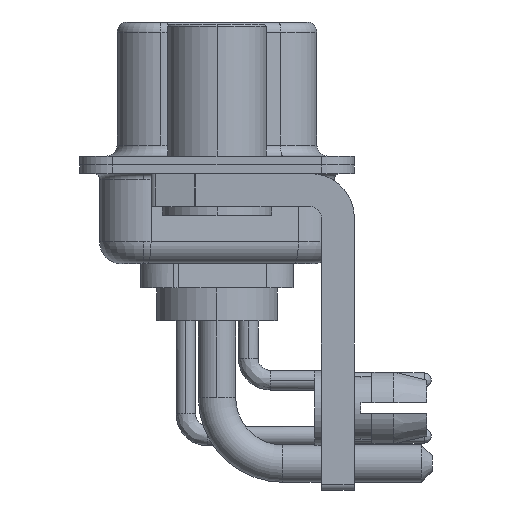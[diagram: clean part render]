
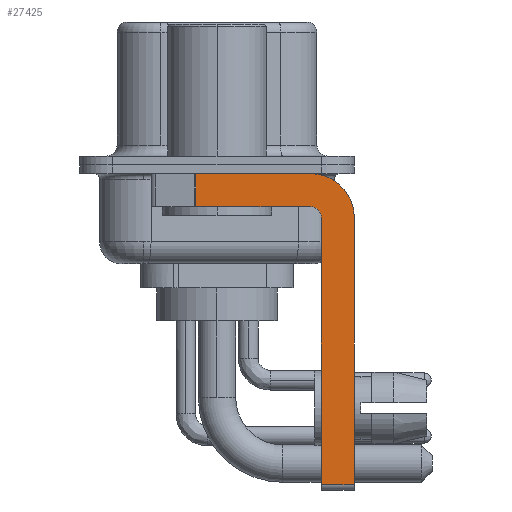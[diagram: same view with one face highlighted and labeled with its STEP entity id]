
A CAD part, left-side view. The second image highlights one B-rep face of the part: STEP entity #27425.
In plain terms, the highlighted planar face has unit normal (-1, 0, 0).
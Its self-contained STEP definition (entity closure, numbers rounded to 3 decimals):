
#953 = CARTESIAN_POINT ( 'NONE',  ( -2.9, -6.25, -2.4 ) ) ;
#1040 = EDGE_CURVE ( 'NONE', #17544, #20139, #19166, .T. ) ;
#1058 = VERTEX_POINT ( 'NONE', #6571 ) ;
#1455 = VERTEX_POINT ( 'NONE', #2155 ) ;
#1502 = LINE ( 'NONE', #8292, #12081 ) ;
#1587 = FACE_OUTER_BOUND ( 'NONE', #15525, .T. ) ;
#2068 = ORIENTED_EDGE ( 'NONE', *, *, #6072, .F. ) ;
#2155 = CARTESIAN_POINT ( 'NONE',  ( -2.9, -6.25, -2.4 ) ) ;
#2426 = EDGE_CURVE ( 'NONE', #4631, #17544, #14822, .T. ) ;
#2539 = CARTESIAN_POINT ( 'NONE',  ( -2.9, 3., -0.4 ) ) ;
#2830 = AXIS2_PLACEMENT_3D ( 'NONE', #15882, #17999, #25402 ) ;
#3077 = LINE ( 'NONE', #23118, #5850 ) ;
#3378 = EDGE_CURVE ( 'NONE', #4631, #26459, #1502, .T. ) ;
#3731 = CARTESIAN_POINT ( 'NONE',  ( -2.9, 0.978, -0.4 ) ) ;
#4164 = DIRECTION ( 'NONE',  ( 1., 0., 0. ) ) ;
#4443 = DIRECTION ( 'NONE',  ( 0., 0., -1. ) ) ;
#4631 = VERTEX_POINT ( 'NONE', #29277 ) ;
#5850 = VECTOR ( 'NONE', #9849, 1000. ) ;
#6072 = EDGE_CURVE ( 'NONE', #20139, #6119, #21003, .T. ) ;
#6119 = VERTEX_POINT ( 'NONE', #27779 ) ;
#6432 = CARTESIAN_POINT ( 'NONE',  ( -2.9, -4.25, -2.4 ) ) ;
#6571 = CARTESIAN_POINT ( 'NONE',  ( -2.9, -4.25, -0.4 ) ) ;
#6691 = CARTESIAN_POINT ( 'NONE',  ( -2.9, -4.75, -2.4 ) ) ;
#6985 = ORIENTED_EDGE ( 'NONE', *, *, #3378, .T. ) ;
#8292 = CARTESIAN_POINT ( 'NONE',  ( -2.9, -4.25, -14.55 ) ) ;
#9143 = ORIENTED_EDGE ( 'NONE', *, *, #14889, .T. ) ;
#9465 = DIRECTION ( 'NONE',  ( 0., -1., 0. ) ) ;
#9836 = ORIENTED_EDGE ( 'NONE', *, *, #1040, .F. ) ;
#9849 = DIRECTION ( 'NONE',  ( 0., 0., -1. ) ) ;
#9856 = CARTESIAN_POINT ( 'NONE',  ( -2.9, -4.25, -1.9 ) ) ;
#10759 = DIRECTION ( 'NONE',  ( 0., 0., 1. ) ) ;
#11224 = ORIENTED_EDGE ( 'NONE', *, *, #2426, .F. ) ;
#11385 = DIRECTION ( 'NONE',  ( 0., 0., -1. ) ) ;
#12081 = VECTOR ( 'NONE', #19882, 1000. ) ;
#12334 = ORIENTED_EDGE ( 'NONE', *, *, #12372, .F. ) ;
#12372 = EDGE_CURVE ( 'NONE', #18295, #1058, #26037, .T. ) ;
#12521 = CARTESIAN_POINT ( 'NONE',  ( -2.9, -4.25, -1.9 ) ) ;
#14790 = DIRECTION ( 'NONE',  ( 0., 0., -1. ) ) ;
#14822 = LINE ( 'NONE', #29266, #29324 ) ;
#14889 = EDGE_CURVE ( 'NONE', #18295, #6119, #3077, .T. ) ;
#15279 = AXIS2_PLACEMENT_3D ( 'NONE', #6432, #4164, #11385 ) ;
#15417 = DIRECTION ( 'NONE',  ( 1., 0., 0. ) ) ;
#15525 = EDGE_LOOP ( 'NONE', ( #12334, #9143, #2068, #9836, #11224, #6985, #21900, #28237 ) ) ;
#15680 = VECTOR ( 'NONE', #14790, 1000. ) ;
#15864 = CARTESIAN_POINT ( 'NONE',  ( -2.9, -4.25, -2.4 ) ) ;
#15882 = CARTESIAN_POINT ( 'NONE',  ( -2.9, -4.25, -2.4 ) ) ;
#17044 = LINE ( 'NONE', #953, #15680 ) ;
#17544 = VERTEX_POINT ( 'NONE', #6691 ) ;
#17999 = DIRECTION ( 'NONE',  ( -1., 0., 0. ) ) ;
#18295 = VERTEX_POINT ( 'NONE', #3731 ) ;
#19165 = AXIS2_PLACEMENT_3D ( 'NONE', #15864, #15417, #4443 ) ;
#19166 = CIRCLE ( 'NONE', #2830, 0.5 ) ;
#19882 = DIRECTION ( 'NONE',  ( 0., -1., 0. ) ) ;
#20139 = VERTEX_POINT ( 'NONE', #12521 ) ;
#21003 = LINE ( 'NONE', #9856, #21878 ) ;
#21878 = VECTOR ( 'NONE', #23731, 1000. ) ;
#21900 = ORIENTED_EDGE ( 'NONE', *, *, #24473, .F. ) ;
#23118 = CARTESIAN_POINT ( 'NONE',  ( -2.9, 0.978, -1.9 ) ) ;
#23731 = DIRECTION ( 'NONE',  ( 0., 1., 0. ) ) ;
#24473 = EDGE_CURVE ( 'NONE', #1455, #26459, #17044, .T. ) ;
#24571 = VECTOR ( 'NONE', #9465, 1000. ) ;
#25402 = DIRECTION ( 'NONE',  ( 0., 0., 1. ) ) ;
#25527 = EDGE_CURVE ( 'NONE', #1058, #1455, #27321, .T. ) ;
#26037 = LINE ( 'NONE', #2539, #24571 ) ;
#26459 = VERTEX_POINT ( 'NONE', #29510 ) ;
#27321 = CIRCLE ( 'NONE', #15279, 2. ) ;
#27338 = PLANE ( 'NONE',  #19165 ) ;
#27425 = ADVANCED_FACE ( 'NONE', ( #1587 ), #27338, .F. ) ;
#27779 = CARTESIAN_POINT ( 'NONE',  ( -2.9, 0.978, -1.9 ) ) ;
#28237 = ORIENTED_EDGE ( 'NONE', *, *, #25527, .F. ) ;
#29266 = CARTESIAN_POINT ( 'NONE',  ( -2.9, -4.75, -14.8 ) ) ;
#29277 = CARTESIAN_POINT ( 'NONE',  ( -2.9, -4.75, -14.55 ) ) ;
#29324 = VECTOR ( 'NONE', #10759, 1000. ) ;
#29510 = CARTESIAN_POINT ( 'NONE',  ( -2.9, -6.25, -14.55 ) ) ;
